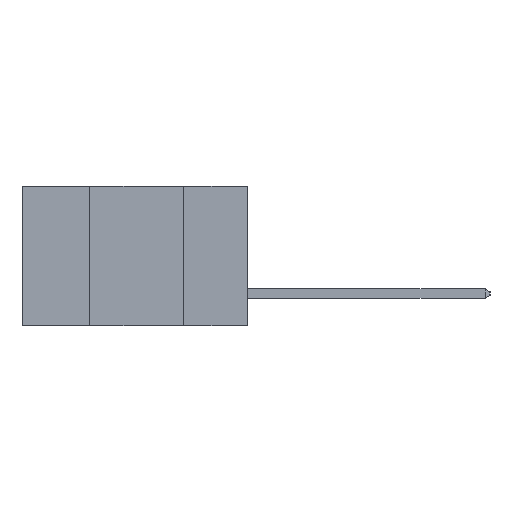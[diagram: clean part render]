
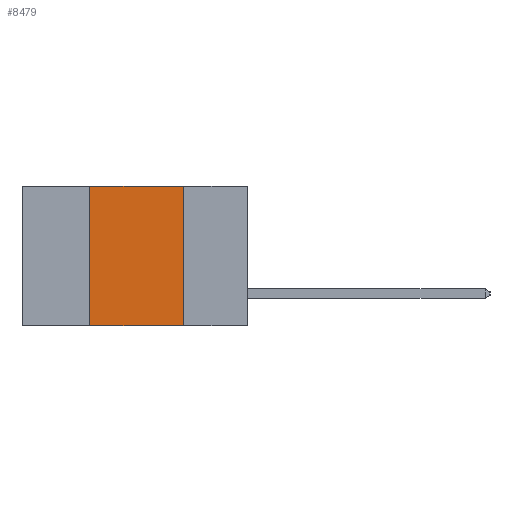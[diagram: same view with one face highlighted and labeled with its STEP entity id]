
A CAD part, left-side view. The second image highlights one B-rep face of the part: STEP entity #8479.
In plain terms, the highlighted planar face has unit normal (-1, 0, 0).
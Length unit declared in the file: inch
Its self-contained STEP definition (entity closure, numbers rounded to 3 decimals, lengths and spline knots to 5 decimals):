
#233 = VECTOR ( 'NONE', #13204, 39.37008 ) ;
#384 = VERTEX_POINT ( 'NONE', #627 ) ;
#627 = CARTESIAN_POINT ( 'NONE',  ( 0., 0.17, -0.37 ) ) ;
#981 = ORIENTED_EDGE ( 'NONE', *, *, #4077, .F. ) ;
#2869 = FACE_OUTER_BOUND ( 'NONE', #9634, .T. ) ;
#3551 = LINE ( 'NONE', #15757, #13403 ) ;
#4077 = EDGE_CURVE ( 'NONE', #12046, #384, #11669, .T. ) ;
#4671 = DIRECTION ( 'NONE',  ( 0., 0., -1. ) ) ;
#5540 = CARTESIAN_POINT ( 'NONE',  ( 0., 0.17, 0. ) ) ;
#5556 = EDGE_CURVE ( 'NONE', #15151, #384, #3551, .T. ) ;
#5693 = AXIS2_PLACEMENT_3D ( 'NONE', #10271, #10981, #14214 ) ;
#5728 = ORIENTED_EDGE ( 'NONE', *, *, #5556, .T. ) ;
#6903 = ORIENTED_EDGE ( 'NONE', *, *, #13905, .F. ) ;
#8223 = LINE ( 'NONE', #8787, #11206 ) ;
#8294 = VECTOR ( 'NONE', #4671, 39.37008 ) ;
#8479 = ADVANCED_FACE ( 'NONE', ( #2869 ), #11205, .F. ) ;
#8787 = CARTESIAN_POINT ( 'NONE',  ( 0., 0.42, 0. ) ) ;
#9347 = CARTESIAN_POINT ( 'NONE',  ( 0., 0.42, -0.37 ) ) ;
#9634 = EDGE_LOOP ( 'NONE', ( #981, #9680, #6903, #5728 ) ) ;
#9680 = ORIENTED_EDGE ( 'NONE', *, *, #14202, .F. ) ;
#10271 = CARTESIAN_POINT ( 'NONE',  ( 0., 0.6, 0. ) ) ;
#10981 = DIRECTION ( 'NONE',  ( 1., 0., 0. ) ) ;
#11205 = PLANE ( 'NONE',  #5693 ) ;
#11206 = VECTOR ( 'NONE', #16338, 39.37008 ) ;
#11669 = LINE ( 'NONE', #5540, #8294 ) ;
#11768 = VERTEX_POINT ( 'NONE', #15949 ) ;
#11938 = CARTESIAN_POINT ( 'NONE',  ( 0., 0.6, 0. ) ) ;
#12046 = VERTEX_POINT ( 'NONE', #15215 ) ;
#13204 = DIRECTION ( 'NONE',  ( 0., -1., 0. ) ) ;
#13403 = VECTOR ( 'NONE', #15142, 39.37008 ) ;
#13558 = LINE ( 'NONE', #11938, #233 ) ;
#13905 = EDGE_CURVE ( 'NONE', #15151, #11768, #8223, .T. ) ;
#14202 = EDGE_CURVE ( 'NONE', #11768, #12046, #13558, .T. ) ;
#14214 = DIRECTION ( 'NONE',  ( 0., 0., -1. ) ) ;
#15142 = DIRECTION ( 'NONE',  ( 0., -1., 0. ) ) ;
#15151 = VERTEX_POINT ( 'NONE', #9347 ) ;
#15215 = CARTESIAN_POINT ( 'NONE',  ( 0., 0.17, 0. ) ) ;
#15757 = CARTESIAN_POINT ( 'NONE',  ( 0., 0.6, -0.37 ) ) ;
#15949 = CARTESIAN_POINT ( 'NONE',  ( 0., 0.42, 0. ) ) ;
#16338 = DIRECTION ( 'NONE',  ( 0., 0., 1. ) ) ;
